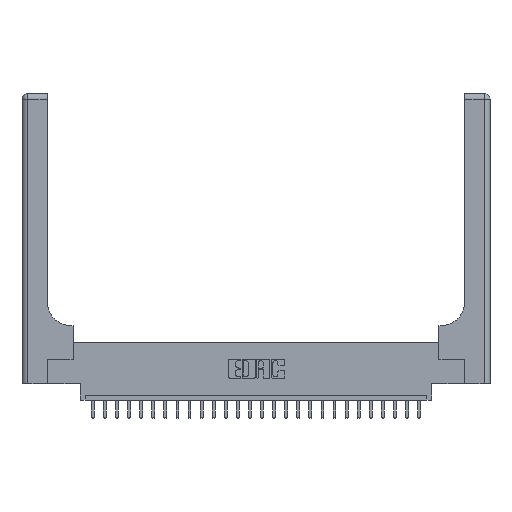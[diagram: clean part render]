
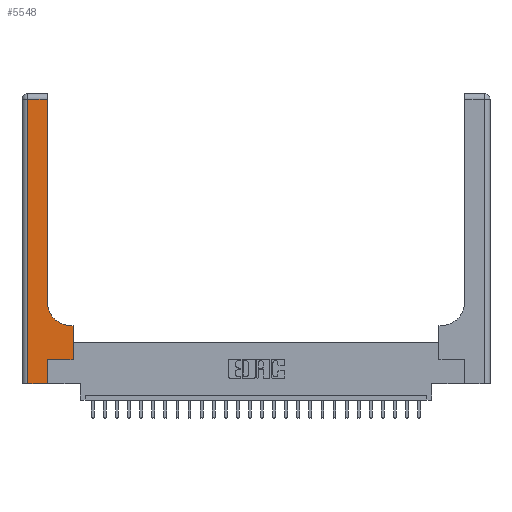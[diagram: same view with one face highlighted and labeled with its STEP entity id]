
A CAD part, top view. The second image highlights one B-rep face of the part: STEP entity #5548.
In plain terms, the highlighted planar face has unit normal (0, 0, 1).
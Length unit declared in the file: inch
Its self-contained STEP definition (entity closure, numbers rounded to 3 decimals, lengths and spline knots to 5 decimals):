
#41 = LINE ( 'NONE', #22124, #18242 ) ;
#160 = ORIENTED_EDGE ( 'NONE', *, *, #20269, .T. ) ;
#704 = LINE ( 'NONE', #7020, #17717 ) ;
#740 = VERTEX_POINT ( 'NONE', #13870 ) ;
#1109 = EDGE_CURVE ( 'NONE', #6025, #1749, #13011, .T. ) ;
#1208 = FACE_OUTER_BOUND ( 'NONE', #19812, .T. ) ;
#1225 = VERTEX_POINT ( 'NONE', #18247 ) ;
#1527 = DIRECTION ( 'NONE',  ( 1., 0., 0. ) ) ;
#1630 = CARTESIAN_POINT ( 'NONE',  ( 0., 3., 0.37 ) ) ;
#1749 = VERTEX_POINT ( 'NONE', #6406 ) ;
#3256 = CIRCLE ( 'NONE', #19838, 0.25 ) ;
#3642 = DIRECTION ( 'NONE',  ( -1., 0., 0. ) ) ;
#4445 = CARTESIAN_POINT ( 'NONE',  ( 0.528, 0.25, 0.37 ) ) ;
#4540 = DIRECTION ( 'NONE',  ( 0., -1., 0. ) ) ;
#5276 = DIRECTION ( 'NONE',  ( 0., 1., 0. ) ) ;
#5548 = ADVANCED_FACE ( 'NONE', ( #1208 ), #7564, .F. ) ;
#6025 = VERTEX_POINT ( 'NONE', #20399 ) ;
#6118 = EDGE_CURVE ( 'NONE', #1225, #11905, #3256, .T. ) ;
#6406 = CARTESIAN_POINT ( 'NONE',  ( 0.06, 0., 0.37 ) ) ;
#6848 = EDGE_CURVE ( 'NONE', #11694, #1225, #14507, .T. ) ;
#6931 = CARTESIAN_POINT ( 'NONE',  ( 0.265, 0., 0.37 ) ) ;
#7020 = CARTESIAN_POINT ( 'NONE',  ( 0.26, 3., 0.37 ) ) ;
#7025 = LINE ( 'NONE', #6931, #14140 ) ;
#7272 = VECTOR ( 'NONE', #15908, 39.37008 ) ;
#7563 = LINE ( 'NONE', #21943, #7272 ) ;
#7564 = PLANE ( 'NONE',  #11539 ) ;
#7970 = VECTOR ( 'NONE', #19041, 39.37008 ) ;
#8249 = VECTOR ( 'NONE', #4540, 39.37008 ) ;
#9146 = CARTESIAN_POINT ( 'NONE',  ( 0.265, 0., 0.37 ) ) ;
#10830 = CARTESIAN_POINT ( 'NONE',  ( 0., 0., 0.37 ) ) ;
#11033 = ORIENTED_EDGE ( 'NONE', *, *, #6118, .T. ) ;
#11480 = VERTEX_POINT ( 'NONE', #4445 ) ;
#11539 = AXIS2_PLACEMENT_3D ( 'NONE', #1630, #24614, #3642 ) ;
#11694 = VERTEX_POINT ( 'NONE', #22871 ) ;
#11905 = VERTEX_POINT ( 'NONE', #18995 ) ;
#12020 = VERTEX_POINT ( 'NONE', #22932 ) ;
#12073 = ORIENTED_EDGE ( 'NONE', *, *, #23360, .T. ) ;
#12415 = VECTOR ( 'NONE', #22889, 39.37008 ) ;
#12750 = DIRECTION ( 'NONE',  ( 0., 0., -1. ) ) ;
#13011 = LINE ( 'NONE', #15975, #8249 ) ;
#13290 = CARTESIAN_POINT ( 'NONE',  ( 0.265, 0.25, 0.37 ) ) ;
#13620 = ORIENTED_EDGE ( 'NONE', *, *, #23194, .T. ) ;
#13870 = CARTESIAN_POINT ( 'NONE',  ( 0.265, 0.25, 0.37 ) ) ;
#14140 = VECTOR ( 'NONE', #18005, 39.37008 ) ;
#14507 = LINE ( 'NONE', #24639, #12415 ) ;
#15908 = DIRECTION ( 'NONE',  ( -1., 0., 0. ) ) ;
#15975 = CARTESIAN_POINT ( 'NONE',  ( 0.06, 3., 0.37 ) ) ;
#16584 = DIRECTION ( 'NONE',  ( 1., 0., 0. ) ) ;
#17420 = ORIENTED_EDGE ( 'NONE', *, *, #6848, .T. ) ;
#17717 = VECTOR ( 'NONE', #5276, 39.37008 ) ;
#17967 = DIRECTION ( 'NONE',  ( 0., 1., 0. ) ) ;
#18005 = DIRECTION ( 'NONE',  ( 0., 1., 0. ) ) ;
#18137 = EDGE_CURVE ( 'NONE', #11480, #11694, #41, .T. ) ;
#18139 = VECTOR ( 'NONE', #16584, 39.37008 ) ;
#18242 = VECTOR ( 'NONE', #17967, 39.37008 ) ;
#18247 = CARTESIAN_POINT ( 'NONE',  ( 0.51, 0.6, 0.37 ) ) ;
#18995 = CARTESIAN_POINT ( 'NONE',  ( 0.26, 0.85, 0.37 ) ) ;
#19041 = DIRECTION ( 'NONE',  ( 1., 0., 0. ) ) ;
#19812 = EDGE_LOOP ( 'NONE', ( #12073, #22046, #21615, #160, #13620, #23967, #20504, #17420, #11033 ) ) ;
#19838 = AXIS2_PLACEMENT_3D ( 'NONE', #24323, #12750, #1527 ) ;
#20269 = EDGE_CURVE ( 'NONE', #1749, #22145, #20539, .T. ) ;
#20399 = CARTESIAN_POINT ( 'NONE',  ( 0.06, 2.94, 0.37 ) ) ;
#20504 = ORIENTED_EDGE ( 'NONE', *, *, #18137, .T. ) ;
#20539 = LINE ( 'NONE', #10830, #18139 ) ;
#21615 = ORIENTED_EDGE ( 'NONE', *, *, #1109, .T. ) ;
#21943 = CARTESIAN_POINT ( 'NONE',  ( 0., 2.94, 0.37 ) ) ;
#22046 = ORIENTED_EDGE ( 'NONE', *, *, #24275, .T. ) ;
#22124 = CARTESIAN_POINT ( 'NONE',  ( 0.528, 0.25, 0.37 ) ) ;
#22145 = VERTEX_POINT ( 'NONE', #9146 ) ;
#22337 = EDGE_CURVE ( 'NONE', #740, #11480, #23709, .T. ) ;
#22871 = CARTESIAN_POINT ( 'NONE',  ( 0.528, 0.6, 0.37 ) ) ;
#22889 = DIRECTION ( 'NONE',  ( -1., 0., 0. ) ) ;
#22932 = CARTESIAN_POINT ( 'NONE',  ( 0.26, 2.94, 0.37 ) ) ;
#23194 = EDGE_CURVE ( 'NONE', #22145, #740, #7025, .T. ) ;
#23360 = EDGE_CURVE ( 'NONE', #11905, #12020, #704, .T. ) ;
#23709 = LINE ( 'NONE', #13290, #7970 ) ;
#23967 = ORIENTED_EDGE ( 'NONE', *, *, #22337, .T. ) ;
#24275 = EDGE_CURVE ( 'NONE', #12020, #6025, #7563, .T. ) ;
#24323 = CARTESIAN_POINT ( 'NONE',  ( 0.51, 0.85, 0.37 ) ) ;
#24614 = DIRECTION ( 'NONE',  ( 0., 0., -1. ) ) ;
#24639 = CARTESIAN_POINT ( 'NONE',  ( 0.26, 0.6, 0.37 ) ) ;
